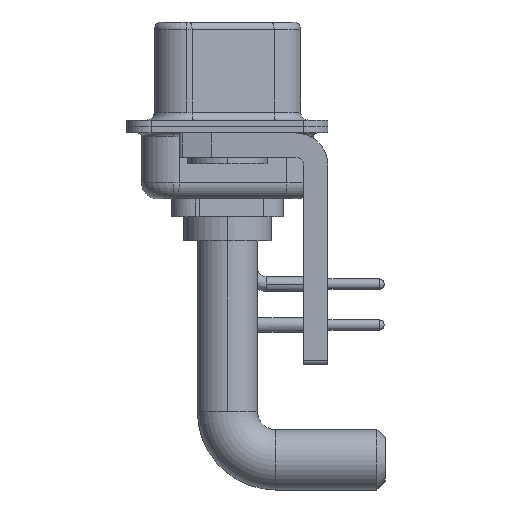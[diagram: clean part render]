
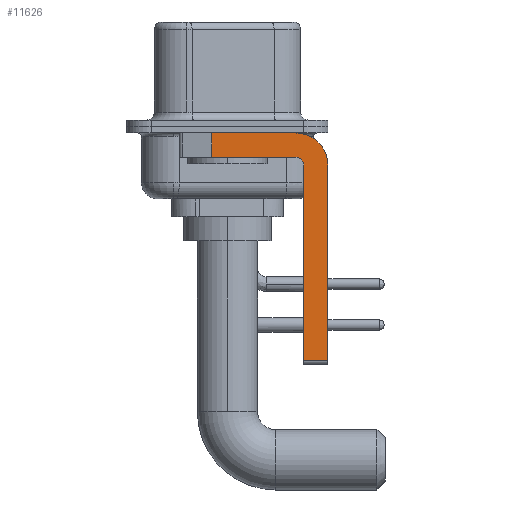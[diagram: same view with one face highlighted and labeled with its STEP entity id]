
A CAD part, left-side view. The second image highlights one B-rep face of the part: STEP entity #11626.
In plain terms, the highlighted planar face has unit normal (-1, 0, 0).
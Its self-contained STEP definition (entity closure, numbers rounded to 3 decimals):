
#307 = EDGE_CURVE ( 'NONE', #7801, #13551, #23666, .T. ) ;
#589 = EDGE_CURVE ( 'NONE', #2976, #13551, #7317, .T. ) ;
#921 = EDGE_CURVE ( 'NONE', #7801, #19887, #1397, .T. ) ;
#1397 = LINE ( 'NONE', #5354, #21009 ) ;
#1488 = ORIENTED_EDGE ( 'NONE', *, *, #589, .F. ) ;
#2610 = CARTESIAN_POINT ( 'NONE',  ( -2.9, -6.25, -2.4 ) ) ;
#2976 = VERTEX_POINT ( 'NONE', #16896 ) ;
#3345 = AXIS2_PLACEMENT_3D ( 'NONE', #24040, #12154, #10368 ) ;
#3399 = LINE ( 'NONE', #13090, #7537 ) ;
#3658 = DIRECTION ( 'NONE',  ( 1., 0., 0. ) ) ;
#3917 = CARTESIAN_POINT ( 'NONE',  ( -2.9, -4.25, -2.4 ) ) ;
#3993 = DIRECTION ( 'NONE',  ( 0., 0., -1. ) ) ;
#4100 = VECTOR ( 'NONE', #6496, 1000. ) ;
#4876 = DIRECTION ( 'NONE',  ( 0., 1., 0. ) ) ;
#5354 = CARTESIAN_POINT ( 'NONE',  ( -2.9, 3., -0.4 ) ) ;
#5583 = DIRECTION ( 'NONE',  ( 0., 0., -1. ) ) ;
#6039 = CARTESIAN_POINT ( 'NONE',  ( -2.9, 0.978, -1.9 ) ) ;
#6496 = DIRECTION ( 'NONE',  ( 0., -1., 0. ) ) ;
#7125 = EDGE_CURVE ( 'NONE', #13676, #24732, #16321, .T. ) ;
#7317 = LINE ( 'NONE', #9097, #24635 ) ;
#7363 = EDGE_CURVE ( 'NONE', #19887, #10006, #24104, .T. ) ;
#7413 = ORIENTED_EDGE ( 'NONE', *, *, #11066, .F. ) ;
#7537 = VECTOR ( 'NONE', #19222, 1000. ) ;
#7801 = VERTEX_POINT ( 'NONE', #18961 ) ;
#7882 = VECTOR ( 'NONE', #14614, 1000. ) ;
#8084 = ORIENTED_EDGE ( 'NONE', *, *, #7363, .F. ) ;
#8443 = ORIENTED_EDGE ( 'NONE', *, *, #7125, .T. ) ;
#9080 = CARTESIAN_POINT ( 'NONE',  ( -2.9, 0.978, -1.9 ) ) ;
#9097 = CARTESIAN_POINT ( 'NONE',  ( -2.9, -4.25, -1.9 ) ) ;
#9460 = FACE_OUTER_BOUND ( 'NONE', #12294, .T. ) ;
#9756 = ORIENTED_EDGE ( 'NONE', *, *, #921, .F. ) ;
#10006 = VERTEX_POINT ( 'NONE', #15483 ) ;
#10086 = EDGE_CURVE ( 'NONE', #16496, #2976, #15577, .T. ) ;
#10368 = DIRECTION ( 'NONE',  ( 0., 0., 1. ) ) ;
#10595 = CARTESIAN_POINT ( 'NONE',  ( -2.9, -4.75, -2.4 ) ) ;
#11066 = EDGE_CURVE ( 'NONE', #10006, #24732, #24455, .T. ) ;
#11626 = ADVANCED_FACE ( 'NONE', ( #9460 ), #15213, .F. ) ;
#12154 = DIRECTION ( 'NONE',  ( -1., 0., 0. ) ) ;
#12294 = EDGE_LOOP ( 'NONE', ( #9756, #14861, #1488, #12651, #23703, #8443, #7413, #8084 ) ) ;
#12400 = CARTESIAN_POINT ( 'NONE',  ( -2.9, -6.25, -14.55 ) ) ;
#12566 = EDGE_CURVE ( 'NONE', #13676, #16496, #3399, .T. ) ;
#12651 = ORIENTED_EDGE ( 'NONE', *, *, #10086, .F. ) ;
#13077 = AXIS2_PLACEMENT_3D ( 'NONE', #3917, #3658, #5583 ) ;
#13090 = CARTESIAN_POINT ( 'NONE',  ( -2.9, -4.75, -14.8 ) ) ;
#13160 = CARTESIAN_POINT ( 'NONE',  ( -2.9, -4.25, -2.4 ) ) ;
#13551 = VERTEX_POINT ( 'NONE', #9080 ) ;
#13676 = VERTEX_POINT ( 'NONE', #15582 ) ;
#14614 = DIRECTION ( 'NONE',  ( 0., 0., -1. ) ) ;
#14836 = DIRECTION ( 'NONE',  ( 0., 0., -1. ) ) ;
#14861 = ORIENTED_EDGE ( 'NONE', *, *, #307, .T. ) ;
#15213 = PLANE ( 'NONE',  #25027 ) ;
#15483 = CARTESIAN_POINT ( 'NONE',  ( -2.9, -6.25, -2.4 ) ) ;
#15577 = CIRCLE ( 'NONE', #3345, 0.5 ) ;
#15582 = CARTESIAN_POINT ( 'NONE',  ( -2.9, -4.75, -14.55 ) ) ;
#16321 = LINE ( 'NONE', #19787, #4100 ) ;
#16496 = VERTEX_POINT ( 'NONE', #10595 ) ;
#16896 = CARTESIAN_POINT ( 'NONE',  ( -2.9, -4.25, -1.9 ) ) ;
#16995 = DIRECTION ( 'NONE',  ( 1., 0., 0. ) ) ;
#17668 = VECTOR ( 'NONE', #3993, 1000. ) ;
#18961 = CARTESIAN_POINT ( 'NONE',  ( -2.9, 0.978, -0.4 ) ) ;
#19222 = DIRECTION ( 'NONE',  ( 0., 0., 1. ) ) ;
#19787 = CARTESIAN_POINT ( 'NONE',  ( -2.9, -4.25, -14.55 ) ) ;
#19887 = VERTEX_POINT ( 'NONE', #25214 ) ;
#20570 = DIRECTION ( 'NONE',  ( 0., -1., 0. ) ) ;
#21009 = VECTOR ( 'NONE', #20570, 1000. ) ;
#23666 = LINE ( 'NONE', #6039, #17668 ) ;
#23703 = ORIENTED_EDGE ( 'NONE', *, *, #12566, .F. ) ;
#24040 = CARTESIAN_POINT ( 'NONE',  ( -2.9, -4.25, -2.4 ) ) ;
#24104 = CIRCLE ( 'NONE', #13077, 2. ) ;
#24455 = LINE ( 'NONE', #2610, #7882 ) ;
#24635 = VECTOR ( 'NONE', #4876, 1000. ) ;
#24732 = VERTEX_POINT ( 'NONE', #12400 ) ;
#25027 = AXIS2_PLACEMENT_3D ( 'NONE', #13160, #16995, #14836 ) ;
#25214 = CARTESIAN_POINT ( 'NONE',  ( -2.9, -4.25, -0.4 ) ) ;
